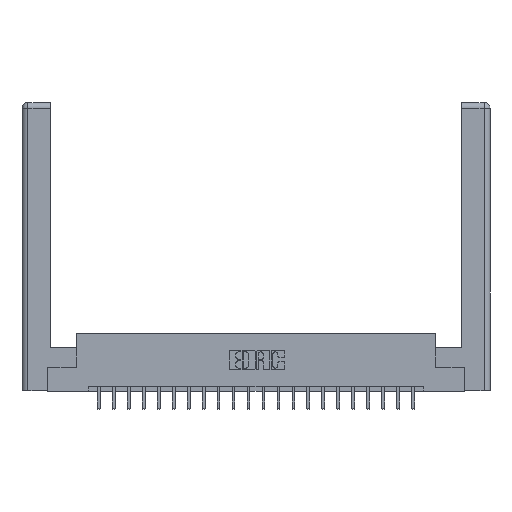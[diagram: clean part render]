
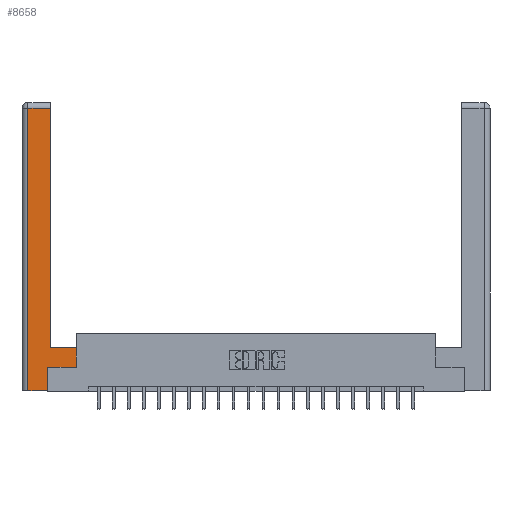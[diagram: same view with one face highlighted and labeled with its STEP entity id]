
A CAD part, top view. The second image highlights one B-rep face of the part: STEP entity #8658.
In plain terms, the highlighted planar face has unit normal (0, 0, 1).
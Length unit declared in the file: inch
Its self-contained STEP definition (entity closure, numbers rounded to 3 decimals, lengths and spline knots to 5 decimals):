
#286 = LINE ( 'NONE', #14992, #21421 ) ;
#427 = CARTESIAN_POINT ( 'NONE',  ( 0.565, 0.45, 0. ) ) ;
#670 = VECTOR ( 'NONE', #2929, 39.37008 ) ;
#705 = ORIENTED_EDGE ( 'NONE', *, *, #1280, .T. ) ;
#1012 = DIRECTION ( 'NONE',  ( 0., 1., 0. ) ) ;
#1122 = CARTESIAN_POINT ( 'NONE',  ( 0., 0., 0. ) ) ;
#1280 = EDGE_CURVE ( 'NONE', #1759, #4696, #1377, .T. ) ;
#1377 = LINE ( 'NONE', #15377, #20353 ) ;
#1575 = CARTESIAN_POINT ( 'NONE',  ( 0.0615, 2.94, 0. ) ) ;
#1759 = VERTEX_POINT ( 'NONE', #13216 ) ;
#2712 = CARTESIAN_POINT ( 'NONE',  ( 0.0615, 0., 0. ) ) ;
#2748 = VECTOR ( 'NONE', #4621, 39.37008 ) ;
#2929 = DIRECTION ( 'NONE',  ( -1., 0., 0. ) ) ;
#3306 = AXIS2_PLACEMENT_3D ( 'NONE', #1122, #13252, #16519 ) ;
#3395 = EDGE_CURVE ( 'NONE', #3838, #11557, #12564, .T. ) ;
#3658 = FACE_OUTER_BOUND ( 'NONE', #11391, .T. ) ;
#3838 = VERTEX_POINT ( 'NONE', #8720 ) ;
#4621 = DIRECTION ( 'NONE',  ( 0., -1., 0. ) ) ;
#4673 = LINE ( 'NONE', #21604, #13337 ) ;
#4696 = VERTEX_POINT ( 'NONE', #1575 ) ;
#5160 = EDGE_CURVE ( 'NONE', #8293, #1759, #4673, .T. ) ;
#5265 = EDGE_CURVE ( 'NONE', #5672, #3838, #286, .T. ) ;
#5672 = VERTEX_POINT ( 'NONE', #20881 ) ;
#5685 = CARTESIAN_POINT ( 'NONE',  ( 0.265, 0., 0. ) ) ;
#6419 = CARTESIAN_POINT ( 'NONE',  ( 0.565, 0.245, 0. ) ) ;
#6570 = CARTESIAN_POINT ( 'NONE',  ( 0.295, 0.45, 0. ) ) ;
#6722 = DIRECTION ( 'NONE',  ( -1., 0., 0. ) ) ;
#7293 = VECTOR ( 'NONE', #15931, 39.37008 ) ;
#7966 = VECTOR ( 'NONE', #10419, 39.37008 ) ;
#8293 = VERTEX_POINT ( 'NONE', #11815 ) ;
#8658 = ADVANCED_FACE ( 'NONE', ( #3658 ), #19914, .F. ) ;
#8720 = CARTESIAN_POINT ( 'NONE',  ( 0.265, 0.245, 0. ) ) ;
#8783 = EDGE_CURVE ( 'NONE', #19343, #8293, #20720, .T. ) ;
#9874 = DIRECTION ( 'NONE',  ( 0., 1., 0. ) ) ;
#10061 = ORIENTED_EDGE ( 'NONE', *, *, #8783, .T. ) ;
#10419 = DIRECTION ( 'NONE',  ( 1., 0., 0. ) ) ;
#10767 = CARTESIAN_POINT ( 'NONE',  ( 0.565, 0.45, 0. ) ) ;
#11066 = ORIENTED_EDGE ( 'NONE', *, *, #19480, .T. ) ;
#11391 = EDGE_LOOP ( 'NONE', ( #13497, #705, #11066, #11899, #18003, #22082, #17264, #10061 ) ) ;
#11557 = VERTEX_POINT ( 'NONE', #13646 ) ;
#11815 = CARTESIAN_POINT ( 'NONE',  ( 0.295, 0.45, 0. ) ) ;
#11899 = ORIENTED_EDGE ( 'NONE', *, *, #16633, .T. ) ;
#12564 = LINE ( 'NONE', #6419, #7966 ) ;
#12788 = VERTEX_POINT ( 'NONE', #14849 ) ;
#13216 = CARTESIAN_POINT ( 'NONE',  ( 0.295, 2.94, 0. ) ) ;
#13252 = DIRECTION ( 'NONE',  ( 0., 0., -1. ) ) ;
#13337 = VECTOR ( 'NONE', #1012, 39.37008 ) ;
#13497 = ORIENTED_EDGE ( 'NONE', *, *, #5160, .T. ) ;
#13646 = CARTESIAN_POINT ( 'NONE',  ( 0.565, 0.245, 0. ) ) ;
#14849 = CARTESIAN_POINT ( 'NONE',  ( 0.0615, 0., 0. ) ) ;
#14992 = CARTESIAN_POINT ( 'NONE',  ( 0.265, 0.245, 0. ) ) ;
#15377 = CARTESIAN_POINT ( 'NONE',  ( 0.0615, 2.94, 0. ) ) ;
#15931 = DIRECTION ( 'NONE',  ( 0., 1., 0. ) ) ;
#16191 = VECTOR ( 'NONE', #19313, 39.37008 ) ;
#16263 = LINE ( 'NONE', #10767, #7293 ) ;
#16325 = LINE ( 'NONE', #2712, #2748 ) ;
#16519 = DIRECTION ( 'NONE',  ( -1., 0., 0. ) ) ;
#16633 = EDGE_CURVE ( 'NONE', #12788, #5672, #20765, .T. ) ;
#17264 = ORIENTED_EDGE ( 'NONE', *, *, #21000, .T. ) ;
#18003 = ORIENTED_EDGE ( 'NONE', *, *, #5265, .T. ) ;
#19313 = DIRECTION ( 'NONE',  ( 1., 0., 0. ) ) ;
#19343 = VERTEX_POINT ( 'NONE', #427 ) ;
#19480 = EDGE_CURVE ( 'NONE', #4696, #12788, #16325, .T. ) ;
#19914 = PLANE ( 'NONE',  #3306 ) ;
#20353 = VECTOR ( 'NONE', #6722, 39.37008 ) ;
#20720 = LINE ( 'NONE', #6570, #670 ) ;
#20765 = LINE ( 'NONE', #5685, #16191 ) ;
#20881 = CARTESIAN_POINT ( 'NONE',  ( 0.265, 0., 0. ) ) ;
#21000 = EDGE_CURVE ( 'NONE', #11557, #19343, #16263, .T. ) ;
#21421 = VECTOR ( 'NONE', #9874, 39.37008 ) ;
#21604 = CARTESIAN_POINT ( 'NONE',  ( 0.295, 3., 0. ) ) ;
#22082 = ORIENTED_EDGE ( 'NONE', *, *, #3395, .T. ) ;
